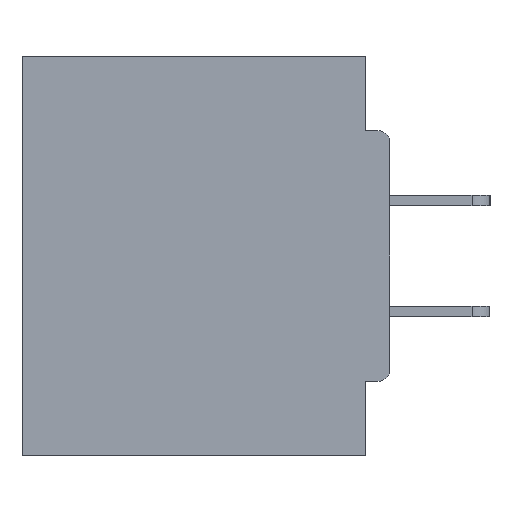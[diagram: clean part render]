
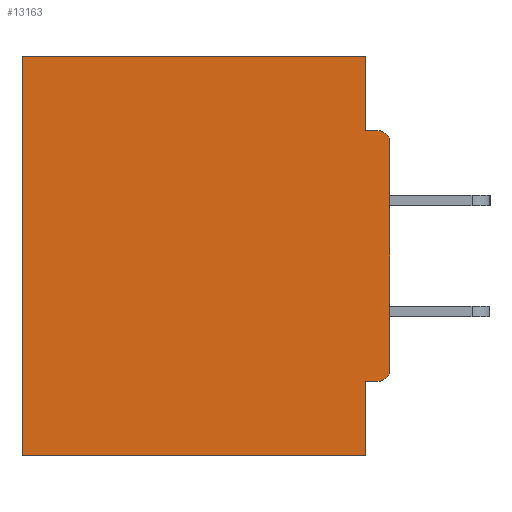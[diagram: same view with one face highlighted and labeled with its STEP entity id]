
A CAD part, left-side view. The second image highlights one B-rep face of the part: STEP entity #13163.
In plain terms, the highlighted planar face has unit normal (-1, 0, 0).
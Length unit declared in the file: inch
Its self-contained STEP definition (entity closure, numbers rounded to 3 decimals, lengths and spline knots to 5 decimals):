
#249 = ORIENTED_EDGE ( 'NONE', *, *, #12714, .F. ) ;
#435 = VECTOR ( 'NONE', #21508, 39.37008 ) ;
#789 = VERTEX_POINT ( 'NONE', #5743 ) ;
#1332 = CARTESIAN_POINT ( 'NONE',  ( 0.298, 0., -0.3915 ) ) ;
#1388 = EDGE_CURVE ( 'NONE', #31583, #12355, #29987, .T. ) ;
#1598 = CARTESIAN_POINT ( 'NONE',  ( 0.298, 0.46, 0. ) ) ;
#1738 = LINE ( 'NONE', #23694, #8685 ) ;
#1928 = LINE ( 'NONE', #2159, #31525 ) ;
#2159 = CARTESIAN_POINT ( 'NONE',  ( 0.298, 0., 0. ) ) ;
#2295 = DIRECTION ( 'NONE',  ( 0., 0., -1. ) ) ;
#2485 = VERTEX_POINT ( 'NONE', #13268 ) ;
#3300 = CARTESIAN_POINT ( 'NONE',  ( 0.298, 0., -0.4065 ) ) ;
#3308 = CARTESIAN_POINT ( 'NONE',  ( 0.298, 0.031, -0.5 ) ) ;
#3343 = VECTOR ( 'NONE', #18577, 39.37008 ) ;
#3426 = CARTESIAN_POINT ( 'NONE',  ( 0.298, 0.015, -0.3915 ) ) ;
#3874 = DIRECTION ( 'NONE',  ( 0., 0., -1. ) ) ;
#4172 = VECTOR ( 'NONE', #3874, 39.37008 ) ;
#5743 = CARTESIAN_POINT ( 'NONE',  ( 0.298, 0., -0.1085 ) ) ;
#7766 = CARTESIAN_POINT ( 'NONE',  ( 0.298, 0., -0.5 ) ) ;
#7977 = DIRECTION ( 'NONE',  ( 0., 1., 0. ) ) ;
#8685 = VECTOR ( 'NONE', #29026, 39.37008 ) ;
#9135 = ORIENTED_EDGE ( 'NONE', *, *, #24470, .T. ) ;
#9982 = DIRECTION ( 'NONE',  ( 0., 1., 0. ) ) ;
#10030 = DIRECTION ( 'NONE',  ( 0., 0., -1. ) ) ;
#10243 = CARTESIAN_POINT ( 'NONE',  ( 0.298, 0.46, 0. ) ) ;
#10660 = LINE ( 'NONE', #10243, #21983 ) ;
#10711 = EDGE_CURVE ( 'NONE', #789, #22602, #24186, .T. ) ;
#10720 = AXIS2_PLACEMENT_3D ( 'NONE', #3426, #19125, #29245 ) ;
#12000 = CARTESIAN_POINT ( 'NONE',  ( 0.298, 0.031, -0.5 ) ) ;
#12355 = VERTEX_POINT ( 'NONE', #23909 ) ;
#12507 = DIRECTION ( 'NONE',  ( 1., 0., 0. ) ) ;
#12714 = EDGE_CURVE ( 'NONE', #30753, #16450, #31330, .T. ) ;
#13163 = ADVANCED_FACE ( 'NONE', ( #13848 ), #14873, .F. ) ;
#13268 = CARTESIAN_POINT ( 'NONE',  ( 0.298, 0.46, -0.5 ) ) ;
#13848 = FACE_OUTER_BOUND ( 'NONE', #27252, .T. ) ;
#14040 = DIRECTION ( 'NONE',  ( 0., 0., -1. ) ) ;
#14112 = EDGE_CURVE ( 'NONE', #30678, #33437, #28794, .T. ) ;
#14873 = PLANE ( 'NONE',  #24355 ) ;
#15118 = ORIENTED_EDGE ( 'NONE', *, *, #26812, .F. ) ;
#15811 = LINE ( 'NONE', #3300, #435 ) ;
#15950 = CARTESIAN_POINT ( 'NONE',  ( 0.298, 0.031, 0. ) ) ;
#16174 = AXIS2_PLACEMENT_3D ( 'NONE', #32195, #24595, #19259 ) ;
#16450 = VERTEX_POINT ( 'NONE', #20975 ) ;
#18577 = DIRECTION ( 'NONE',  ( 0., -1., 0. ) ) ;
#18941 = CARTESIAN_POINT ( 'NONE',  ( 0.298, 0.015, -0.0935 ) ) ;
#19125 = DIRECTION ( 'NONE',  ( -1., 0., 0. ) ) ;
#19259 = DIRECTION ( 'NONE',  ( 0., 0., -1. ) ) ;
#19262 = EDGE_CURVE ( 'NONE', #21658, #2485, #10660, .T. ) ;
#20975 = CARTESIAN_POINT ( 'NONE',  ( 0.298, 0.031, -0.5 ) ) ;
#21508 = DIRECTION ( 'NONE',  ( 0., 1., 0. ) ) ;
#21658 = VERTEX_POINT ( 'NONE', #1598 ) ;
#21888 = EDGE_CURVE ( 'NONE', #30678, #30753, #15811, .T. ) ;
#21983 = VECTOR ( 'NONE', #2295, 39.37008 ) ;
#22554 = VECTOR ( 'NONE', #7977, 39.37008 ) ;
#22602 = VERTEX_POINT ( 'NONE', #18941 ) ;
#23165 = ORIENTED_EDGE ( 'NONE', *, *, #27517, .F. ) ;
#23636 = ORIENTED_EDGE ( 'NONE', *, *, #21888, .F. ) ;
#23694 = CARTESIAN_POINT ( 'NONE',  ( 0.298, 0., 0. ) ) ;
#23909 = CARTESIAN_POINT ( 'NONE',  ( 0.298, 0.031, -0.0935 ) ) ;
#24186 = CIRCLE ( 'NONE', #16174, 0.015 ) ;
#24355 = AXIS2_PLACEMENT_3D ( 'NONE', #25533, #12507, #10030 ) ;
#24470 = EDGE_CURVE ( 'NONE', #31583, #21658, #1928, .T. ) ;
#24595 = DIRECTION ( 'NONE',  ( -1., 0., 0. ) ) ;
#24665 = VECTOR ( 'NONE', #14040, 39.37008 ) ;
#24812 = LINE ( 'NONE', #31522, #3343 ) ;
#25533 = CARTESIAN_POINT ( 'NONE',  ( 0.298, 0., 0. ) ) ;
#26812 = EDGE_CURVE ( 'NONE', #789, #33437, #1738, .T. ) ;
#27252 = EDGE_LOOP ( 'NONE', ( #29148, #23165, #30320, #9135, #33467, #30340, #249, #23636, #27881, #15118 ) ) ;
#27517 = EDGE_CURVE ( 'NONE', #12355, #22602, #24812, .T. ) ;
#27881 = ORIENTED_EDGE ( 'NONE', *, *, #14112, .T. ) ;
#28078 = EDGE_CURVE ( 'NONE', #16450, #2485, #29084, .T. ) ;
#28794 = CIRCLE ( 'NONE', #10720, 0.015 ) ;
#29026 = DIRECTION ( 'NONE',  ( 0., 0., -1. ) ) ;
#29084 = LINE ( 'NONE', #7766, #22554 ) ;
#29148 = ORIENTED_EDGE ( 'NONE', *, *, #10711, .T. ) ;
#29245 = DIRECTION ( 'NONE',  ( 0., 0., -1. ) ) ;
#29987 = LINE ( 'NONE', #3308, #24665 ) ;
#30320 = ORIENTED_EDGE ( 'NONE', *, *, #1388, .F. ) ;
#30340 = ORIENTED_EDGE ( 'NONE', *, *, #28078, .F. ) ;
#30678 = VERTEX_POINT ( 'NONE', #32239 ) ;
#30753 = VERTEX_POINT ( 'NONE', #32990 ) ;
#31330 = LINE ( 'NONE', #12000, #4172 ) ;
#31522 = CARTESIAN_POINT ( 'NONE',  ( 0.298, 0., -0.0935 ) ) ;
#31525 = VECTOR ( 'NONE', #9982, 39.37008 ) ;
#31583 = VERTEX_POINT ( 'NONE', #15950 ) ;
#32195 = CARTESIAN_POINT ( 'NONE',  ( 0.298, 0.015, -0.1085 ) ) ;
#32239 = CARTESIAN_POINT ( 'NONE',  ( 0.298, 0.015, -0.4065 ) ) ;
#32990 = CARTESIAN_POINT ( 'NONE',  ( 0.298, 0.031, -0.4065 ) ) ;
#33437 = VERTEX_POINT ( 'NONE', #1332 ) ;
#33467 = ORIENTED_EDGE ( 'NONE', *, *, #19262, .T. ) ;
